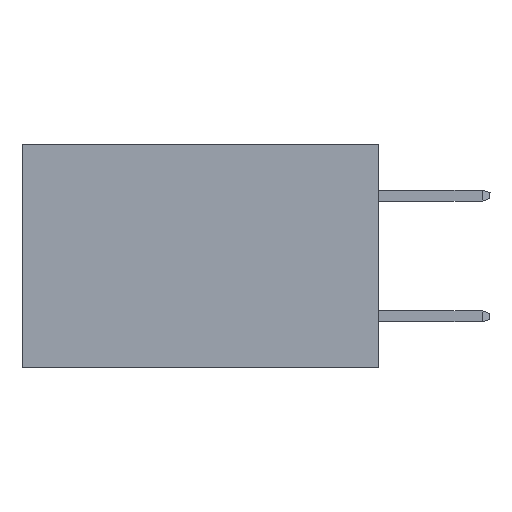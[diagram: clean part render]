
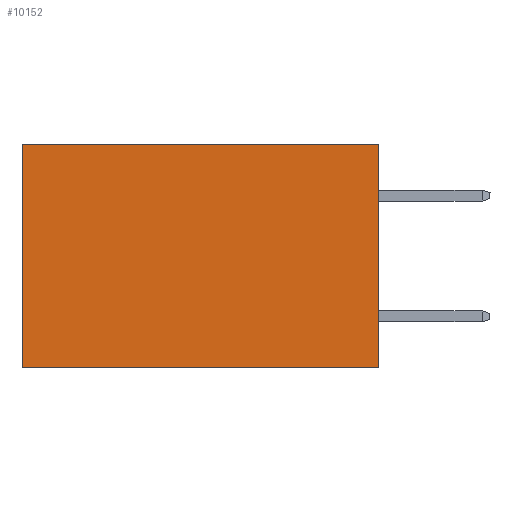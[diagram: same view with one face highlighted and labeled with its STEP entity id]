
A CAD part, left-side view. The second image highlights one B-rep face of the part: STEP entity #10152.
In plain terms, the highlighted planar face has unit normal (-1, 0, 0).
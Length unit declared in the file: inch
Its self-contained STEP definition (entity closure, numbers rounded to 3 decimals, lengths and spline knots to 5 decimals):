
#58 = VERTEX_POINT ( 'NONE', #1685 ) ;
#578 = CARTESIAN_POINT ( 'NONE',  ( 0.277, 0., 0. ) ) ;
#905 = CARTESIAN_POINT ( 'NONE',  ( 0.277, 0., -0.37 ) ) ;
#1348 = ORIENTED_EDGE ( 'NONE', *, *, #9461, .T. ) ;
#1685 = CARTESIAN_POINT ( 'NONE',  ( 0.277, 0.59, -0.37 ) ) ;
#1688 = VECTOR ( 'NONE', #8288, 39.37008 ) ;
#1751 = FACE_OUTER_BOUND ( 'NONE', #6681, .T. ) ;
#1891 = CARTESIAN_POINT ( 'NONE',  ( 0.277, 0., -0.37 ) ) ;
#1910 = LINE ( 'NONE', #6267, #2679 ) ;
#2026 = VERTEX_POINT ( 'NONE', #578 ) ;
#2264 = ORIENTED_EDGE ( 'NONE', *, *, #7120, .F. ) ;
#2436 = DIRECTION ( 'NONE',  ( 0., 0., -1. ) ) ;
#2679 = VECTOR ( 'NONE', #10071, 39.37008 ) ;
#3414 = DIRECTION ( 'NONE',  ( 0., 1., 0. ) ) ;
#4392 = LINE ( 'NONE', #905, #10070 ) ;
#4575 = ORIENTED_EDGE ( 'NONE', *, *, #6760, .T. ) ;
#4971 = VECTOR ( 'NONE', #6714, 39.37008 ) ;
#5302 = CARTESIAN_POINT ( 'NONE',  ( 0.277, 0.59, 0. ) ) ;
#5534 = AXIS2_PLACEMENT_3D ( 'NONE', #5643, #7208, #2436 ) ;
#5643 = CARTESIAN_POINT ( 'NONE',  ( 0.277, 0., -0.37 ) ) ;
#6100 = VERTEX_POINT ( 'NONE', #8825 ) ;
#6267 = CARTESIAN_POINT ( 'NONE',  ( 0.277, 0., 0. ) ) ;
#6681 = EDGE_LOOP ( 'NONE', ( #4575, #2264, #9061, #1348 ) ) ;
#6714 = DIRECTION ( 'NONE',  ( 0., 0., -1. ) ) ;
#6760 = EDGE_CURVE ( 'NONE', #9296, #58, #9840, .T. ) ;
#6820 = LINE ( 'NONE', #1891, #4971 ) ;
#7120 = EDGE_CURVE ( 'NONE', #6100, #58, #4392, .T. ) ;
#7208 = DIRECTION ( 'NONE',  ( 1., 0., 0. ) ) ;
#8288 = DIRECTION ( 'NONE',  ( 0., 0., -1. ) ) ;
#8825 = CARTESIAN_POINT ( 'NONE',  ( 0.277, 0., -0.37 ) ) ;
#9061 = ORIENTED_EDGE ( 'NONE', *, *, #9160, .F. ) ;
#9160 = EDGE_CURVE ( 'NONE', #2026, #6100, #6820, .T. ) ;
#9296 = VERTEX_POINT ( 'NONE', #5302 ) ;
#9461 = EDGE_CURVE ( 'NONE', #2026, #9296, #1910, .T. ) ;
#9823 = CARTESIAN_POINT ( 'NONE',  ( 0.277, 0.59, -0.37 ) ) ;
#9840 = LINE ( 'NONE', #9823, #1688 ) ;
#10070 = VECTOR ( 'NONE', #3414, 39.37008 ) ;
#10071 = DIRECTION ( 'NONE',  ( 0., 1., 0. ) ) ;
#10152 = ADVANCED_FACE ( 'NONE', ( #1751 ), #10253, .F. ) ;
#10253 = PLANE ( 'NONE',  #5534 ) ;
